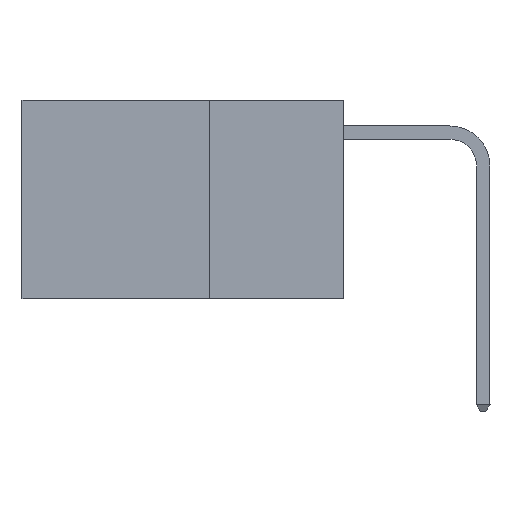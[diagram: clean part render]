
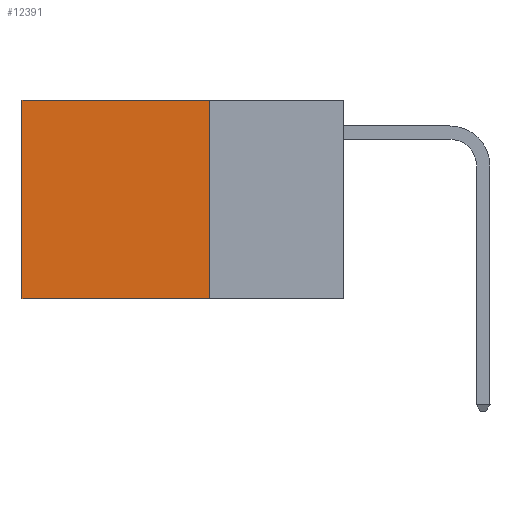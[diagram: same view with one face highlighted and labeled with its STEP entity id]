
A CAD part, left-side view. The second image highlights one B-rep face of the part: STEP entity #12391.
In plain terms, the highlighted planar face has unit normal (-1, 0, 0).
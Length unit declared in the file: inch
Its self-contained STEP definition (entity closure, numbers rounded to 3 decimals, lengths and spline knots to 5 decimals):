
#146 = VECTOR ( 'NONE', #1244, 39.37008 ) ;
#248 = VECTOR ( 'NONE', #438, 39.37008 ) ;
#269 = LINE ( 'NONE', #482, #248 ) ;
#438 = DIRECTION ( 'NONE',  ( 0., 1., 0. ) ) ;
#482 = CARTESIAN_POINT ( 'NONE',  ( 0.2625, 0.25, 0. ) ) ;
#1244 = DIRECTION ( 'NONE',  ( 0., 1., 0. ) ) ;
#2288 = AXIS2_PLACEMENT_3D ( 'NONE', #15836, #17086, #9338 ) ;
#2559 = VERTEX_POINT ( 'NONE', #8167 ) ;
#2782 = ORIENTED_EDGE ( 'NONE', *, *, #15650, .T. ) ;
#3216 = ORIENTED_EDGE ( 'NONE', *, *, #10576, .F. ) ;
#4832 = CARTESIAN_POINT ( 'NONE',  ( 0.2625, 0.6, -0.37 ) ) ;
#5700 = VECTOR ( 'NONE', #7808, 39.37008 ) ;
#6959 = EDGE_CURVE ( 'NONE', #8983, #9736, #269, .T. ) ;
#7808 = DIRECTION ( 'NONE',  ( 0., 0., -1. ) ) ;
#7956 = VECTOR ( 'NONE', #11829, 39.37008 ) ;
#7996 = CARTESIAN_POINT ( 'NONE',  ( 0.2625, 0.25, -0.37 ) ) ;
#8132 = EDGE_LOOP ( 'NONE', ( #2782, #3216, #15820, #11849 ) ) ;
#8167 = CARTESIAN_POINT ( 'NONE',  ( 0.2625, 0.25, -0.37 ) ) ;
#8454 = CARTESIAN_POINT ( 'NONE',  ( 0.2625, 0.25, 0. ) ) ;
#8983 = VERTEX_POINT ( 'NONE', #8454 ) ;
#9338 = DIRECTION ( 'NONE',  ( 0., 0., -1. ) ) ;
#9736 = VERTEX_POINT ( 'NONE', #11198 ) ;
#10523 = CARTESIAN_POINT ( 'NONE',  ( 0.2625, 0.25, 0. ) ) ;
#10576 = EDGE_CURVE ( 'NONE', #2559, #10979, #14705, .T. ) ;
#10979 = VERTEX_POINT ( 'NONE', #4832 ) ;
#11198 = CARTESIAN_POINT ( 'NONE',  ( 0.2625, 0.6, 0. ) ) ;
#11392 = FACE_OUTER_BOUND ( 'NONE', #8132, .T. ) ;
#11829 = DIRECTION ( 'NONE',  ( 0., 0., -1. ) ) ;
#11849 = ORIENTED_EDGE ( 'NONE', *, *, #6959, .T. ) ;
#12391 = ADVANCED_FACE ( 'NONE', ( #11392 ), #14521, .F. ) ;
#12590 = LINE ( 'NONE', #15548, #5700 ) ;
#13917 = EDGE_CURVE ( 'NONE', #8983, #2559, #14811, .T. ) ;
#14521 = PLANE ( 'NONE',  #2288 ) ;
#14705 = LINE ( 'NONE', #7996, #146 ) ;
#14811 = LINE ( 'NONE', #10523, #7956 ) ;
#15548 = CARTESIAN_POINT ( 'NONE',  ( 0.2625, 0.6, 0. ) ) ;
#15650 = EDGE_CURVE ( 'NONE', #9736, #10979, #12590, .T. ) ;
#15820 = ORIENTED_EDGE ( 'NONE', *, *, #13917, .F. ) ;
#15836 = CARTESIAN_POINT ( 'NONE',  ( 0.2625, 0.25, 0. ) ) ;
#17086 = DIRECTION ( 'NONE',  ( 1., 0., 0. ) ) ;
